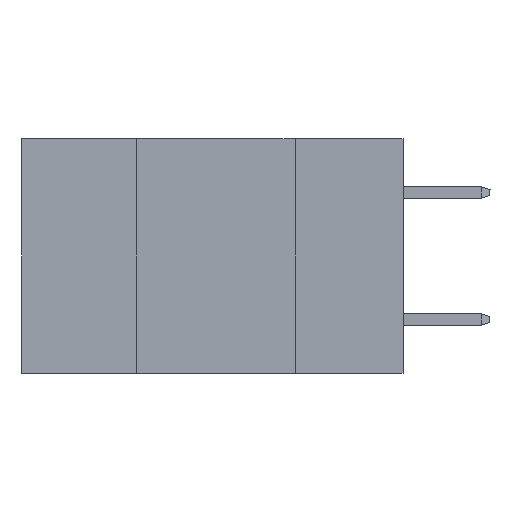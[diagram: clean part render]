
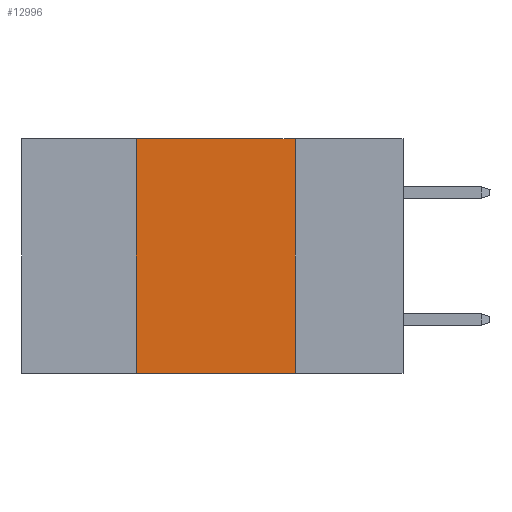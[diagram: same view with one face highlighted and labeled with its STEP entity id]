
A CAD part, left-side view. The second image highlights one B-rep face of the part: STEP entity #12996.
In plain terms, the highlighted planar face has unit normal (-1, 0, 0).
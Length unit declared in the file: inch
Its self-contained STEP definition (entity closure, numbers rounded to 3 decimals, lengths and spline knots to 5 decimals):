
#44 = EDGE_CURVE ( 'NONE', #15760, #19857, #6051, .T. ) ;
#328 = CARTESIAN_POINT ( 'NONE',  ( 0., 0.42, -0.37 ) ) ;
#405 = VECTOR ( 'NONE', #15253, 39.37008 ) ;
#1156 = EDGE_CURVE ( 'NONE', #19857, #9846, #15132, .T. ) ;
#4530 = LINE ( 'NONE', #7914, #17896 ) ;
#5993 = PLANE ( 'NONE',  #13478 ) ;
#6051 = LINE ( 'NONE', #15727, #8021 ) ;
#7781 = VECTOR ( 'NONE', #15630, 39.37008 ) ;
#7842 = LINE ( 'NONE', #13666, #7781 ) ;
#7914 = CARTESIAN_POINT ( 'NONE',  ( 0., 0.6, -0.37 ) ) ;
#8021 = VECTOR ( 'NONE', #22784, 39.37008 ) ;
#9540 = CARTESIAN_POINT ( 'NONE',  ( 0., 0.6, 0. ) ) ;
#9846 = VERTEX_POINT ( 'NONE', #18277 ) ;
#9973 = CARTESIAN_POINT ( 'NONE',  ( 0., 0.6, 0. ) ) ;
#9986 = DIRECTION ( 'NONE',  ( 0., -1., 0. ) ) ;
#10682 = ORIENTED_EDGE ( 'NONE', *, *, #44, .F. ) ;
#12996 = ADVANCED_FACE ( 'NONE', ( #13718 ), #5993, .F. ) ;
#13439 = ORIENTED_EDGE ( 'NONE', *, *, #22986, .F. ) ;
#13478 = AXIS2_PLACEMENT_3D ( 'NONE', #9973, #21157, #17291 ) ;
#13666 = CARTESIAN_POINT ( 'NONE',  ( 0., 0.17, 0. ) ) ;
#13718 = FACE_OUTER_BOUND ( 'NONE', #22016, .T. ) ;
#13756 = ORIENTED_EDGE ( 'NONE', *, *, #1156, .F. ) ;
#14930 = CARTESIAN_POINT ( 'NONE',  ( 0., 0.42, 0. ) ) ;
#15132 = LINE ( 'NONE', #9540, #405 ) ;
#15253 = DIRECTION ( 'NONE',  ( 0., -1., 0. ) ) ;
#15630 = DIRECTION ( 'NONE',  ( 0., 0., -1. ) ) ;
#15727 = CARTESIAN_POINT ( 'NONE',  ( 0., 0.42, 0. ) ) ;
#15760 = VERTEX_POINT ( 'NONE', #328 ) ;
#17291 = DIRECTION ( 'NONE',  ( 0., 0., -1. ) ) ;
#17896 = VECTOR ( 'NONE', #9986, 39.37008 ) ;
#18277 = CARTESIAN_POINT ( 'NONE',  ( 0., 0.17, 0. ) ) ;
#19857 = VERTEX_POINT ( 'NONE', #14930 ) ;
#20544 = VERTEX_POINT ( 'NONE', #23824 ) ;
#21157 = DIRECTION ( 'NONE',  ( 1., 0., 0. ) ) ;
#21587 = ORIENTED_EDGE ( 'NONE', *, *, #23454, .T. ) ;
#22016 = EDGE_LOOP ( 'NONE', ( #13439, #13756, #10682, #21587 ) ) ;
#22784 = DIRECTION ( 'NONE',  ( 0., 0., 1. ) ) ;
#22986 = EDGE_CURVE ( 'NONE', #9846, #20544, #7842, .T. ) ;
#23454 = EDGE_CURVE ( 'NONE', #15760, #20544, #4530, .T. ) ;
#23824 = CARTESIAN_POINT ( 'NONE',  ( 0., 0.17, -0.37 ) ) ;
